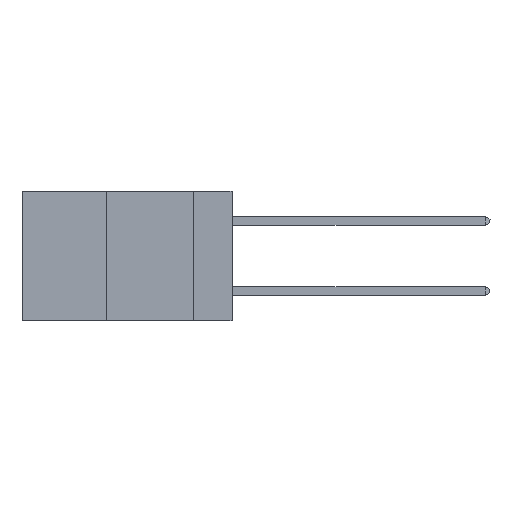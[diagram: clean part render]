
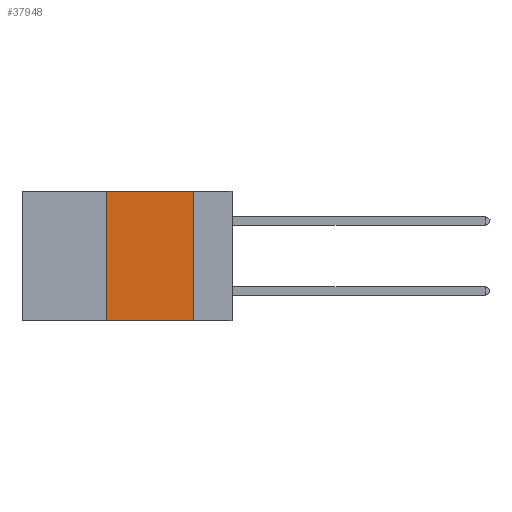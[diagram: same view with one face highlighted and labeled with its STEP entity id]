
A CAD part, left-side view. The second image highlights one B-rep face of the part: STEP entity #37948.
In plain terms, the highlighted planar face has unit normal (-1, 0, 0).
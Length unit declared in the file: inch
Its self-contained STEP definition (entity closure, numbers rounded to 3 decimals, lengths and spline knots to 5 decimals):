
#167 = DIRECTION ( 'NONE',  ( 0., -1., 0. ) ) ;
#333 = CARTESIAN_POINT ( 'NONE',  ( 0., 0.6, -0.37 ) ) ;
#3699 = FACE_OUTER_BOUND ( 'NONE', #29302, .T. ) ;
#8960 = CARTESIAN_POINT ( 'NONE',  ( 0., 0.36, 0. ) ) ;
#11520 = PLANE ( 'NONE',  #33109 ) ;
#11878 = CARTESIAN_POINT ( 'NONE',  ( 0., 0.11, -0.37 ) ) ;
#12951 = CARTESIAN_POINT ( 'NONE',  ( 0., 0.36, -0.37 ) ) ;
#13245 = LINE ( 'NONE', #25281, #39854 ) ;
#14680 = EDGE_CURVE ( 'NONE', #39150, #34652, #13245, .T. ) ;
#15482 = DIRECTION ( 'NONE',  ( 0., 0., -1. ) ) ;
#15741 = VERTEX_POINT ( 'NONE', #12951 ) ;
#15825 = EDGE_CURVE ( 'NONE', #15741, #42288, #21042, .T. ) ;
#16599 = VECTOR ( 'NONE', #167, 39.37008 ) ;
#16805 = CARTESIAN_POINT ( 'NONE',  ( 0., 0.36, 0. ) ) ;
#17576 = CARTESIAN_POINT ( 'NONE',  ( 0., 0.6, 0. ) ) ;
#17818 = ORIENTED_EDGE ( 'NONE', *, *, #26324, .T. ) ;
#18965 = CARTESIAN_POINT ( 'NONE',  ( 0., 0.6, 0. ) ) ;
#21042 = LINE ( 'NONE', #8960, #44085 ) ;
#21636 = CARTESIAN_POINT ( 'NONE',  ( 0., 0.11, 0. ) ) ;
#21892 = ORIENTED_EDGE ( 'NONE', *, *, #15825, .F. ) ;
#22548 = VECTOR ( 'NONE', #28690, 39.37008 ) ;
#24154 = ORIENTED_EDGE ( 'NONE', *, *, #28592, .F. ) ;
#24878 = ORIENTED_EDGE ( 'NONE', *, *, #14680, .F. ) ;
#25281 = CARTESIAN_POINT ( 'NONE',  ( 0., 0.11, 0. ) ) ;
#26324 = EDGE_CURVE ( 'NONE', #15741, #34652, #42653, .T. ) ;
#28592 = EDGE_CURVE ( 'NONE', #42288, #39150, #45602, .T. ) ;
#28690 = DIRECTION ( 'NONE',  ( 0., -1., 0. ) ) ;
#29302 = EDGE_LOOP ( 'NONE', ( #24878, #24154, #21892, #17818 ) ) ;
#30714 = DIRECTION ( 'NONE',  ( 1., 0., 0. ) ) ;
#31466 = DIRECTION ( 'NONE',  ( 0., 0., 1. ) ) ;
#33109 = AXIS2_PLACEMENT_3D ( 'NONE', #18965, #30714, #15482 ) ;
#34652 = VERTEX_POINT ( 'NONE', #11878 ) ;
#36853 = DIRECTION ( 'NONE',  ( 0., 0., -1. ) ) ;
#37948 = ADVANCED_FACE ( 'NONE', ( #3699 ), #11520, .F. ) ;
#39150 = VERTEX_POINT ( 'NONE', #21636 ) ;
#39854 = VECTOR ( 'NONE', #36853, 39.37008 ) ;
#42288 = VERTEX_POINT ( 'NONE', #16805 ) ;
#42653 = LINE ( 'NONE', #333, #16599 ) ;
#44085 = VECTOR ( 'NONE', #31466, 39.37008 ) ;
#45602 = LINE ( 'NONE', #17576, #22548 ) ;
